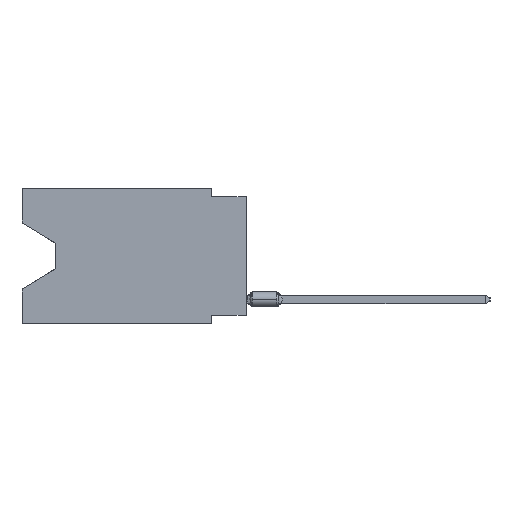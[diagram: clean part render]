
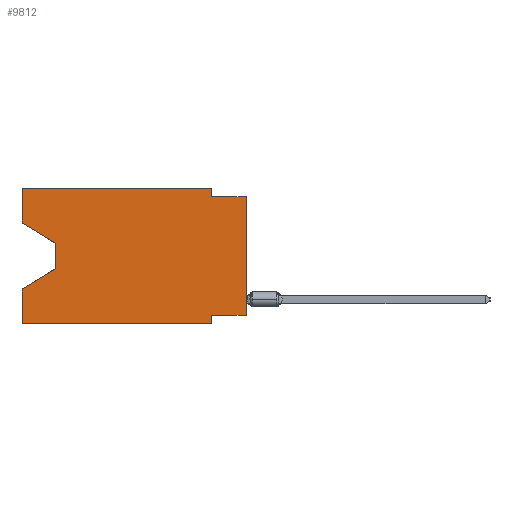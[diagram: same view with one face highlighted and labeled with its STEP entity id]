
A CAD part, left-side view. The second image highlights one B-rep face of the part: STEP entity #9812.
In plain terms, the highlighted planar face has unit normal (-1, 0, 0).
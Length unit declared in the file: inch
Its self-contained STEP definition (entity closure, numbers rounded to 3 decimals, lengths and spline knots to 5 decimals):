
#930 = VERTEX_POINT ( 'NONE', #29600 ) ;
#1400 = CARTESIAN_POINT ( 'NONE',  ( 0., 0.1, 0. ) ) ;
#2123 = VECTOR ( 'NONE', #19641, 39.37008 ) ;
#2548 = LINE ( 'NONE', #24549, #37941 ) ;
#2838 = CARTESIAN_POINT ( 'NONE',  ( 0., 0.1, 0. ) ) ;
#3967 = EDGE_CURVE ( 'NONE', #28849, #18155, #33202, .T. ) ;
#4713 = EDGE_CURVE ( 'NONE', #930, #18155, #23953, .T. ) ;
#4732 = VECTOR ( 'NONE', #27696, 39.37008 ) ;
#6598 = EDGE_CURVE ( 'NONE', #13614, #18104, #39874, .T. ) ;
#6995 = ORIENTED_EDGE ( 'NONE', *, *, #6598, .F. ) ;
#7460 = EDGE_CURVE ( 'NONE', #25033, #11954, #2548, .T. ) ;
#8280 = VECTOR ( 'NONE', #14309, 39.37008 ) ;
#8461 = CARTESIAN_POINT ( 'NONE',  ( 0., 0.1, -0.39 ) ) ;
#8520 = VECTOR ( 'NONE', #21405, 39.37008 ) ;
#9203 = CARTESIAN_POINT ( 'NONE',  ( 0., 0.55, -0.158 ) ) ;
#9213 = ORIENTED_EDGE ( 'NONE', *, *, #14001, .F. ) ;
#9582 = CARTESIAN_POINT ( 'NONE',  ( 0., 0.645, -0.10025 ) ) ;
#9681 = EDGE_CURVE ( 'NONE', #28849, #11954, #16700, .T. ) ;
#9812 = ADVANCED_FACE ( 'NONE', ( #39270 ), #26665, .F. ) ;
#11224 = EDGE_CURVE ( 'NONE', #18104, #12055, #16851, .T. ) ;
#11628 = ORIENTED_EDGE ( 'NONE', *, *, #7460, .T. ) ;
#11743 = EDGE_CURVE ( 'NONE', #38712, #13614, #30255, .T. ) ;
#11894 = DIRECTION ( 'NONE',  ( 0., 0.855, -0.519 ) ) ;
#11954 = VERTEX_POINT ( 'NONE', #34476 ) ;
#12055 = VERTEX_POINT ( 'NONE', #26947 ) ;
#12744 = CARTESIAN_POINT ( 'NONE',  ( 0., 0., -0.025 ) ) ;
#13456 = ORIENTED_EDGE ( 'NONE', *, *, #4713, .F. ) ;
#13614 = VERTEX_POINT ( 'NONE', #27609 ) ;
#13836 = ORIENTED_EDGE ( 'NONE', *, *, #19895, .T. ) ;
#14001 = EDGE_CURVE ( 'NONE', #12055, #21622, #27558, .T. ) ;
#14309 = DIRECTION ( 'NONE',  ( 0., -1., 0. ) ) ;
#14372 = CARTESIAN_POINT ( 'NONE',  ( 0., 0.645, -0.39 ) ) ;
#14690 = CARTESIAN_POINT ( 'NONE',  ( 0., 0.645, -0.39 ) ) ;
#14858 = ORIENTED_EDGE ( 'NONE', *, *, #18907, .T. ) ;
#16700 = LINE ( 'NONE', #25682, #17353 ) ;
#16851 = LINE ( 'NONE', #1400, #21896 ) ;
#17180 = LINE ( 'NONE', #39147, #2123 ) ;
#17196 = LINE ( 'NONE', #9203, #19603 ) ;
#17353 = VECTOR ( 'NONE', #35624, 39.37008 ) ;
#17894 = LINE ( 'NONE', #33375, #19549 ) ;
#18049 = EDGE_CURVE ( 'NONE', #21371, #930, #17894, .T. ) ;
#18094 = DIRECTION ( 'NONE',  ( 0., 1., 0. ) ) ;
#18104 = VERTEX_POINT ( 'NONE', #2838 ) ;
#18155 = VERTEX_POINT ( 'NONE', #28486 ) ;
#18331 = LINE ( 'NONE', #9582, #33304 ) ;
#18907 = EDGE_CURVE ( 'NONE', #30657, #25033, #17196, .T. ) ;
#18927 = DIRECTION ( 'NONE',  ( 0., -0.855, -0.519 ) ) ;
#19549 = VECTOR ( 'NONE', #18094, 39.37008 ) ;
#19603 = VECTOR ( 'NONE', #26562, 39.37008 ) ;
#19641 = DIRECTION ( 'NONE',  ( 0., 0., 1. ) ) ;
#19895 = EDGE_CURVE ( 'NONE', #21371, #21622, #17180, .T. ) ;
#20567 = CARTESIAN_POINT ( 'NONE',  ( 0., 0.645, 0. ) ) ;
#20887 = DIRECTION ( 'NONE',  ( 0., 0., -1. ) ) ;
#21371 = VERTEX_POINT ( 'NONE', #29071 ) ;
#21405 = DIRECTION ( 'NONE',  ( 0., -1., 0. ) ) ;
#21622 = VERTEX_POINT ( 'NONE', #12744 ) ;
#21896 = VECTOR ( 'NONE', #35379, 39.37008 ) ;
#22181 = ORIENTED_EDGE ( 'NONE', *, *, #3967, .T. ) ;
#23953 = LINE ( 'NONE', #8461, #26847 ) ;
#24022 = ORIENTED_EDGE ( 'NONE', *, *, #18049, .F. ) ;
#24549 = CARTESIAN_POINT ( 'NONE',  ( 0., 0.55, -0.232 ) ) ;
#25033 = VERTEX_POINT ( 'NONE', #27072 ) ;
#25682 = CARTESIAN_POINT ( 'NONE',  ( 0., 0.645, 0. ) ) ;
#26562 = DIRECTION ( 'NONE',  ( 0., 0., -1. ) ) ;
#26665 = PLANE ( 'NONE',  #40104 ) ;
#26707 = CARTESIAN_POINT ( 'NONE',  ( 0., 0.55, -0.158 ) ) ;
#26847 = VECTOR ( 'NONE', #20887, 39.37008 ) ;
#26890 = ORIENTED_EDGE ( 'NONE', *, *, #33631, .T. ) ;
#26947 = CARTESIAN_POINT ( 'NONE',  ( 0., 0.1, -0.025 ) ) ;
#27072 = CARTESIAN_POINT ( 'NONE',  ( 0., 0.55, -0.232 ) ) ;
#27558 = LINE ( 'NONE', #29799, #8280 ) ;
#27609 = CARTESIAN_POINT ( 'NONE',  ( 0., 0.645, 0. ) ) ;
#27696 = DIRECTION ( 'NONE',  ( 0., -1., 0. ) ) ;
#28486 = CARTESIAN_POINT ( 'NONE',  ( 0., 0.1, -0.39 ) ) ;
#28849 = VERTEX_POINT ( 'NONE', #14372 ) ;
#29071 = CARTESIAN_POINT ( 'NONE',  ( 0., 0., -0.365 ) ) ;
#29600 = CARTESIAN_POINT ( 'NONE',  ( 0., 0.1, -0.365 ) ) ;
#29799 = CARTESIAN_POINT ( 'NONE',  ( 0., 0., -0.025 ) ) ;
#30255 = LINE ( 'NONE', #33080, #33218 ) ;
#30535 = CARTESIAN_POINT ( 'NONE',  ( 0., 0.645, 0. ) ) ;
#30657 = VERTEX_POINT ( 'NONE', #26707 ) ;
#32197 = ORIENTED_EDGE ( 'NONE', *, *, #11224, .F. ) ;
#33080 = CARTESIAN_POINT ( 'NONE',  ( 0., 0.645, 0. ) ) ;
#33202 = LINE ( 'NONE', #14690, #8520 ) ;
#33218 = VECTOR ( 'NONE', #39183, 39.37008 ) ;
#33304 = VECTOR ( 'NONE', #18927, 39.37008 ) ;
#33375 = CARTESIAN_POINT ( 'NONE',  ( 0., 0., -0.365 ) ) ;
#33631 = EDGE_CURVE ( 'NONE', #38712, #30657, #18331, .T. ) ;
#34476 = CARTESIAN_POINT ( 'NONE',  ( 0., 0.645, -0.28975 ) ) ;
#35099 = CARTESIAN_POINT ( 'NONE',  ( 0., 0.645, -0.10025 ) ) ;
#35379 = DIRECTION ( 'NONE',  ( 0., 0., -1. ) ) ;
#35624 = DIRECTION ( 'NONE',  ( 0., 0., 1. ) ) ;
#35816 = DIRECTION ( 'NONE',  ( 0., 0., -1. ) ) ;
#36022 = DIRECTION ( 'NONE',  ( 1., 0., 0. ) ) ;
#37941 = VECTOR ( 'NONE', #11894, 39.37008 ) ;
#38575 = ORIENTED_EDGE ( 'NONE', *, *, #9681, .F. ) ;
#38712 = VERTEX_POINT ( 'NONE', #35099 ) ;
#39147 = CARTESIAN_POINT ( 'NONE',  ( 0., 0., 0. ) ) ;
#39183 = DIRECTION ( 'NONE',  ( 0., 0., 1. ) ) ;
#39270 = FACE_OUTER_BOUND ( 'NONE', #40214, .T. ) ;
#39874 = LINE ( 'NONE', #30535, #4732 ) ;
#39988 = ORIENTED_EDGE ( 'NONE', *, *, #11743, .F. ) ;
#40104 = AXIS2_PLACEMENT_3D ( 'NONE', #20567, #36022, #35816 ) ;
#40214 = EDGE_LOOP ( 'NONE', ( #26890, #14858, #11628, #38575, #22181, #13456, #24022, #13836, #9213, #32197, #6995, #39988 ) ) ;
